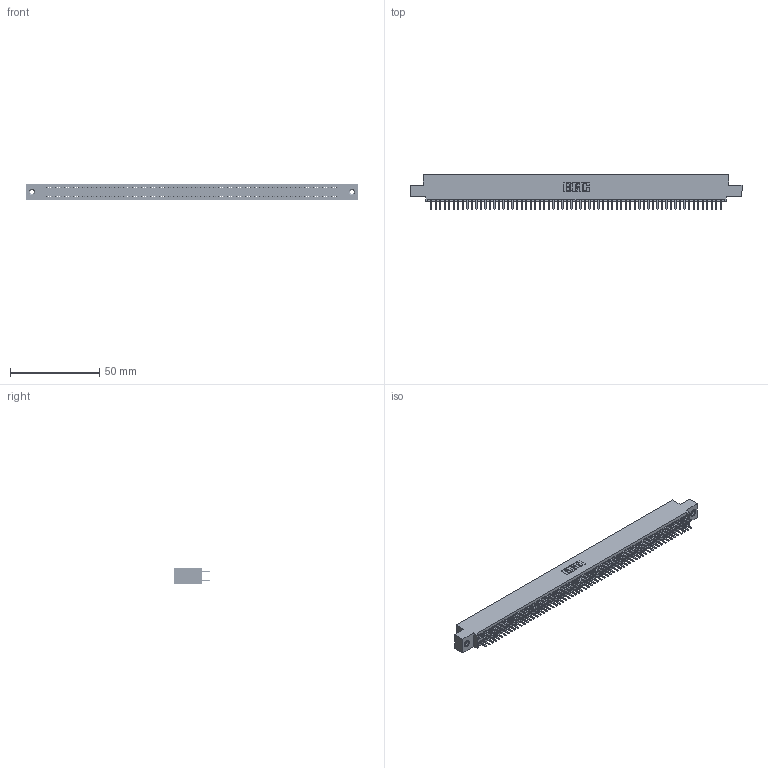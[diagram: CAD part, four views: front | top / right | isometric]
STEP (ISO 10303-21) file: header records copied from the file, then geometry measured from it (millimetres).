
FILE_DESCRIPTION (( 'STEP AP203' ), '1' );
FILE_NAME ('345-130-520-508.STEP', '2018-10-19T23:02:17', ( '' ), ( '' ), 'SwSTEP 2.0', 'SolidWorks 2016', '' );
FILE_SCHEMA (( 'CONFIG_CONTROL_DESIGN' ));
Length unit declared in the file: inch
Products named in the file (4): 345-292-001_345-293-120; 345-250-001_345-250-003-102; 345 Part_0.110 Offset - 0.156 Dia-TI; 345-130-520-508
Assembly tree (133 placements, depth 2):
  345-130-520-508
    345 Part_0.110 Offset - 0.156 Dia-TI
    345-292-001_345-293-120  x130
    345-250-001_345-250-003-102  x2
Bounding box: 186.31 x 19.68 x 9.4 mm (x, y, z)
Volume: 18174.7 mm3; surface area: 27295.4 mm2
Topology: 133 solids, 133 shells, 7210 faces, 20899 edges, 13578 vertices
Faces by surface type: plane 4666, cylinder 2528, cone 12, torus 4
Entity records: 49336 total; most frequent: CARTESIAN_POINT 8243, ORIENTED_EDGE 8158, DIRECTION 7253, EDGE_CURVE 4079, LINE 3663, VECTOR 3663, VERTEX_POINT 2712, AXIS2_PLACEMENT_3D 1795
